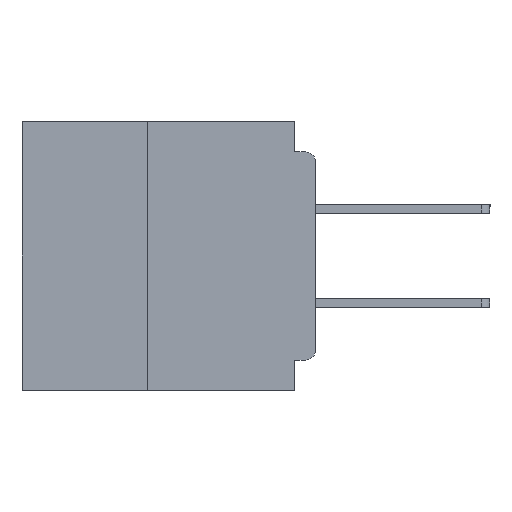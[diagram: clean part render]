
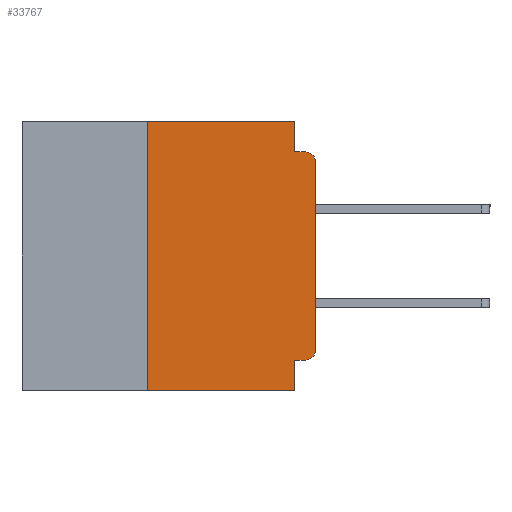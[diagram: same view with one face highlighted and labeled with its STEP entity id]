
A CAD part, left-side view. The second image highlights one B-rep face of the part: STEP entity #33767.
In plain terms, the highlighted planar face has unit normal (-1, 0, 0).
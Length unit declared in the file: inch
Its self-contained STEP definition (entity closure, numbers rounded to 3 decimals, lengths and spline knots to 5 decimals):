
#112 = LINE ( 'NONE', #43142, #9079 ) ;
#537 = CARTESIAN_POINT ( 'NONE',  ( 0., 0., 0. ) ) ;
#762 = AXIS2_PLACEMENT_3D ( 'NONE', #39979, #20050, #43266 ) ;
#1595 = EDGE_CURVE ( 'NONE', #6335, #10838, #6324, .T. ) ;
#1864 = LINE ( 'NONE', #29493, #9726 ) ;
#2148 = CARTESIAN_POINT ( 'NONE',  ( 0., 0.015, -0.045 ) ) ;
#3115 = LINE ( 'NONE', #33826, #37648 ) ;
#3223 = ORIENTED_EDGE ( 'NONE', *, *, #20885, .T. ) ;
#3667 = CARTESIAN_POINT ( 'NONE',  ( 0., 0.015, -0.34 ) ) ;
#4218 = CARTESIAN_POINT ( 'NONE',  ( 0., 0.031, -0.355 ) ) ;
#4597 = CARTESIAN_POINT ( 'NONE',  ( 0., 0.031, 0. ) ) ;
#4851 = CARTESIAN_POINT ( 'NONE',  ( 0., 0.437, 0. ) ) ;
#4975 = LINE ( 'NONE', #36989, #30613 ) ;
#6324 = LINE ( 'NONE', #7787, #23076 ) ;
#6335 = VERTEX_POINT ( 'NONE', #19268 ) ;
#6487 = DIRECTION ( 'NONE',  ( 0., -1., 0. ) ) ;
#6757 = ORIENTED_EDGE ( 'NONE', *, *, #20399, .T. ) ;
#7045 = DIRECTION ( 'NONE',  ( 0., 1., 0. ) ) ;
#7052 = DIRECTION ( 'NONE',  ( 0., 0., -1. ) ) ;
#7787 = CARTESIAN_POINT ( 'NONE',  ( 0., 0.437, 0. ) ) ;
#8215 = DIRECTION ( 'NONE',  ( 0., 0., -1. ) ) ;
#8705 = VECTOR ( 'NONE', #42341, 39.37008 ) ;
#9079 = VECTOR ( 'NONE', #36523, 39.37008 ) ;
#9423 = DIRECTION ( 'NONE',  ( 0., 0., 1. ) ) ;
#9457 = EDGE_CURVE ( 'NONE', #36147, #11623, #21103, .T. ) ;
#9726 = VECTOR ( 'NONE', #9423, 39.37008 ) ;
#9839 = ORIENTED_EDGE ( 'NONE', *, *, #9457, .T. ) ;
#10207 = EDGE_LOOP ( 'NONE', ( #6757, #3223, #40700, #23603, #10723, #18091, #18194, #12097, #31150, #9839 ) ) ;
#10435 = DIRECTION ( 'NONE',  ( 0., -1., 0. ) ) ;
#10723 = ORIENTED_EDGE ( 'NONE', *, *, #1595, .F. ) ;
#10838 = VERTEX_POINT ( 'NONE', #4597 ) ;
#11623 = VERTEX_POINT ( 'NONE', #41627 ) ;
#12090 = VECTOR ( 'NONE', #16164, 39.37008 ) ;
#12097 = ORIENTED_EDGE ( 'NONE', *, *, #38174, .F. ) ;
#14181 = AXIS2_PLACEMENT_3D ( 'NONE', #3667, #27104, #7052 ) ;
#14305 = AXIS2_PLACEMENT_3D ( 'NONE', #4851, #28263, #8215 ) ;
#15319 = EDGE_CURVE ( 'NONE', #10838, #34618, #35371, .T. ) ;
#16164 = DIRECTION ( 'NONE',  ( 0., 0., -1. ) ) ;
#16806 = EDGE_CURVE ( 'NONE', #34618, #35810, #112, .T. ) ;
#18091 = ORIENTED_EDGE ( 'NONE', *, *, #34706, .F. ) ;
#18194 = ORIENTED_EDGE ( 'NONE', *, *, #19699, .T. ) ;
#18230 = CIRCLE ( 'NONE', #762, 0.015 ) ;
#19268 = CARTESIAN_POINT ( 'NONE',  ( 0., 0.25, 0. ) ) ;
#19640 = VERTEX_POINT ( 'NONE', #43307 ) ;
#19699 = EDGE_CURVE ( 'NONE', #35842, #24394, #3115, .T. ) ;
#19982 = LINE ( 'NONE', #22958, #12090 ) ;
#20050 = DIRECTION ( 'NONE',  ( -1., 0., 0. ) ) ;
#20399 = EDGE_CURVE ( 'NONE', #11623, #19640, #29256, .T. ) ;
#20885 = EDGE_CURVE ( 'NONE', #19640, #35810, #18230, .T. ) ;
#21103 = CIRCLE ( 'NONE', #14181, 0.015 ) ;
#22432 = CARTESIAN_POINT ( 'NONE',  ( 0., 0.031, 0. ) ) ;
#22901 = CARTESIAN_POINT ( 'NONE',  ( 0., 0.031, -0.4 ) ) ;
#22958 = CARTESIAN_POINT ( 'NONE',  ( 0., 0.031, -0.4 ) ) ;
#23076 = VECTOR ( 'NONE', #6487, 39.37008 ) ;
#23603 = ORIENTED_EDGE ( 'NONE', *, *, #15319, .F. ) ;
#24394 = VERTEX_POINT ( 'NONE', #22901 ) ;
#27104 = DIRECTION ( 'NONE',  ( -1., 0., 0. ) ) ;
#27172 = VECTOR ( 'NONE', #30741, 39.37008 ) ;
#28263 = DIRECTION ( 'NONE',  ( 1., 0., 0. ) ) ;
#29256 = LINE ( 'NONE', #537, #27172 ) ;
#29493 = CARTESIAN_POINT ( 'NONE',  ( 0., 0.25, -0.4 ) ) ;
#30613 = VECTOR ( 'NONE', #7045, 39.37008 ) ;
#30741 = DIRECTION ( 'NONE',  ( 0., 0., 1. ) ) ;
#30828 = CARTESIAN_POINT ( 'NONE',  ( 0., 0.015, -0.355 ) ) ;
#31150 = ORIENTED_EDGE ( 'NONE', *, *, #35471, .F. ) ;
#31666 = VERTEX_POINT ( 'NONE', #4218 ) ;
#33767 = ADVANCED_FACE ( 'NONE', ( #34402 ), #41477, .F. ) ;
#33826 = CARTESIAN_POINT ( 'NONE',  ( 0., 0.437, -0.4 ) ) ;
#34402 = FACE_OUTER_BOUND ( 'NONE', #10207, .T. ) ;
#34618 = VERTEX_POINT ( 'NONE', #39079 ) ;
#34706 = EDGE_CURVE ( 'NONE', #35842, #6335, #1864, .T. ) ;
#35371 = LINE ( 'NONE', #22432, #8705 ) ;
#35471 = EDGE_CURVE ( 'NONE', #36147, #31666, #4975, .T. ) ;
#35810 = VERTEX_POINT ( 'NONE', #2148 ) ;
#35842 = VERTEX_POINT ( 'NONE', #42447 ) ;
#36147 = VERTEX_POINT ( 'NONE', #30828 ) ;
#36523 = DIRECTION ( 'NONE',  ( 0., -1., 0. ) ) ;
#36989 = CARTESIAN_POINT ( 'NONE',  ( 0., 0., -0.355 ) ) ;
#37648 = VECTOR ( 'NONE', #10435, 39.37008 ) ;
#38174 = EDGE_CURVE ( 'NONE', #31666, #24394, #19982, .T. ) ;
#39079 = CARTESIAN_POINT ( 'NONE',  ( 0., 0.031, -0.045 ) ) ;
#39979 = CARTESIAN_POINT ( 'NONE',  ( 0., 0.015, -0.06 ) ) ;
#40700 = ORIENTED_EDGE ( 'NONE', *, *, #16806, .F. ) ;
#41477 = PLANE ( 'NONE',  #14305 ) ;
#41627 = CARTESIAN_POINT ( 'NONE',  ( 0., 0., -0.34 ) ) ;
#42341 = DIRECTION ( 'NONE',  ( 0., 0., -1. ) ) ;
#42447 = CARTESIAN_POINT ( 'NONE',  ( 0., 0.25, -0.4 ) ) ;
#43142 = CARTESIAN_POINT ( 'NONE',  ( 0., 0., -0.045 ) ) ;
#43266 = DIRECTION ( 'NONE',  ( 0., 0., -1. ) ) ;
#43307 = CARTESIAN_POINT ( 'NONE',  ( 0., 0., -0.06 ) ) ;
